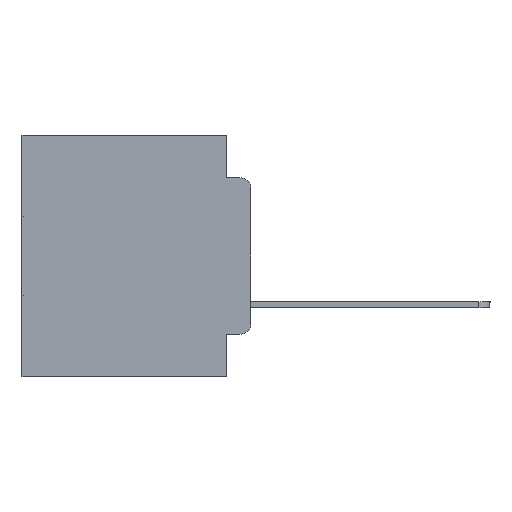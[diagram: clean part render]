
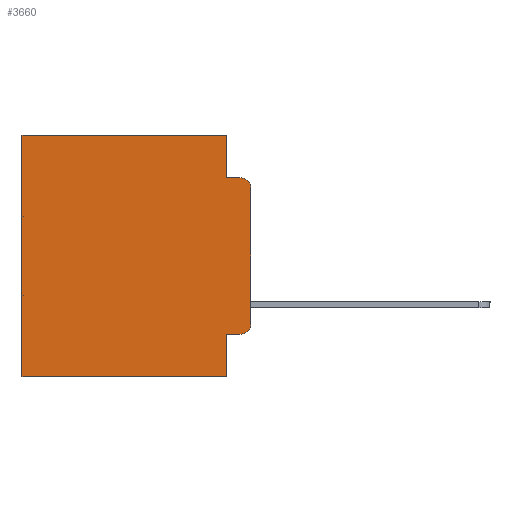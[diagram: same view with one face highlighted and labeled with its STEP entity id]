
A CAD part, left-side view. The second image highlights one B-rep face of the part: STEP entity #3660.
In plain terms, the highlighted planar face has unit normal (-1, 0, 0).
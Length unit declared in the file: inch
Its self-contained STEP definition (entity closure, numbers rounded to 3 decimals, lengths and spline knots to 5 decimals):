
#218 = DIRECTION ( 'NONE',  ( 0., -1., 0. ) ) ;
#1203 = EDGE_CURVE ( 'NONE', #16348, #26457, #9020, .T. ) ;
#1427 = FACE_OUTER_BOUND ( 'NONE', #21408, .T. ) ;
#1746 = VERTEX_POINT ( 'NONE', #16600 ) ;
#1847 = CARTESIAN_POINT ( 'NONE',  ( 0.298, 0.473, 0. ) ) ;
#1998 = ORIENTED_EDGE ( 'NONE', *, *, #12314, .T. ) ;
#2050 = PLANE ( 'NONE',  #3455 ) ;
#2650 = VERTEX_POINT ( 'NONE', #5294 ) ;
#2804 = VECTOR ( 'NONE', #5925, 39.37008 ) ;
#3455 = AXIS2_PLACEMENT_3D ( 'NONE', #23412, #21355, #13927 ) ;
#3605 = DIRECTION ( 'NONE',  ( -1., 0., 0. ) ) ;
#3660 = ADVANCED_FACE ( 'NONE', ( #1427 ), #2050, .F. ) ;
#5294 = CARTESIAN_POINT ( 'NONE',  ( 0.298, 0.02, -0.0885 ) ) ;
#5925 = DIRECTION ( 'NONE',  ( 0., 0., -1. ) ) ;
#5948 = DIRECTION ( 'NONE',  ( -1., 0., 0. ) ) ;
#6258 = DIRECTION ( 'NONE',  ( 0., 0., -1. ) ) ;
#6486 = EDGE_CURVE ( 'NONE', #21719, #12941, #17036, .T. ) ;
#6664 = EDGE_CURVE ( 'NONE', #25098, #12713, #27475, .T. ) ;
#7265 = ORIENTED_EDGE ( 'NONE', *, *, #10635, .F. ) ;
#8189 = ORIENTED_EDGE ( 'NONE', *, *, #6664, .F. ) ;
#8225 = ORIENTED_EDGE ( 'NONE', *, *, #14018, .T. ) ;
#8260 = LINE ( 'NONE', #17913, #14005 ) ;
#8399 = CARTESIAN_POINT ( 'NONE',  ( 0.298, 0.051, 0. ) ) ;
#8950 = CARTESIAN_POINT ( 'NONE',  ( 0.298, 0.02, -0.1085 ) ) ;
#9020 = LINE ( 'NONE', #8399, #13879 ) ;
#9315 = ORIENTED_EDGE ( 'NONE', *, *, #1203, .F. ) ;
#9660 = LINE ( 'NONE', #28969, #24577 ) ;
#10124 = EDGE_CURVE ( 'NONE', #18295, #1746, #8260, .T. ) ;
#10198 = VERTEX_POINT ( 'NONE', #21042 ) ;
#10420 = AXIS2_PLACEMENT_3D ( 'NONE', #15810, #3605, #25456 ) ;
#10635 = EDGE_CURVE ( 'NONE', #26457, #12941, #21210, .T. ) ;
#10666 = CARTESIAN_POINT ( 'NONE',  ( 0.298, 0.051, 0. ) ) ;
#11536 = VECTOR ( 'NONE', #17351, 39.37008 ) ;
#11693 = CARTESIAN_POINT ( 'NONE',  ( 0.298, 0., -0.5 ) ) ;
#11803 = DIRECTION ( 'NONE',  ( 0., 0., -1. ) ) ;
#12004 = ORIENTED_EDGE ( 'NONE', *, *, #31243, .F. ) ;
#12314 = EDGE_CURVE ( 'NONE', #10198, #1746, #20119, .T. ) ;
#12427 = LINE ( 'NONE', #22096, #11536 ) ;
#12503 = ORIENTED_EDGE ( 'NONE', *, *, #10124, .F. ) ;
#12713 = VERTEX_POINT ( 'NONE', #15618 ) ;
#12941 = VERTEX_POINT ( 'NONE', #16563 ) ;
#13879 = VECTOR ( 'NONE', #25955, 39.37008 ) ;
#13927 = DIRECTION ( 'NONE',  ( 0., 0., -1. ) ) ;
#14005 = VECTOR ( 'NONE', #15704, 39.37008 ) ;
#14018 = EDGE_CURVE ( 'NONE', #18295, #2650, #20139, .T. ) ;
#14651 = CARTESIAN_POINT ( 'NONE',  ( 0.298, 0.051, -0.0885 ) ) ;
#15618 = CARTESIAN_POINT ( 'NONE',  ( 0.298, 0.051, -0.0885 ) ) ;
#15704 = DIRECTION ( 'NONE',  ( 0., 0., -1. ) ) ;
#15810 = CARTESIAN_POINT ( 'NONE',  ( 0.298, 0.02, -0.3915 ) ) ;
#16348 = VERTEX_POINT ( 'NONE', #23513 ) ;
#16563 = CARTESIAN_POINT ( 'NONE',  ( 0.298, 0.473, -0.5 ) ) ;
#16600 = CARTESIAN_POINT ( 'NONE',  ( 0.298, 0., -0.3915 ) ) ;
#16622 = VECTOR ( 'NONE', #218, 39.37008 ) ;
#17036 = LINE ( 'NONE', #1847, #17962 ) ;
#17154 = CARTESIAN_POINT ( 'NONE',  ( 0.298, 0., -0.1085 ) ) ;
#17351 = DIRECTION ( 'NONE',  ( 0., -1., 0. ) ) ;
#17738 = DIRECTION ( 'NONE',  ( 0., 1., 0. ) ) ;
#17913 = CARTESIAN_POINT ( 'NONE',  ( 0.298, 0., 0. ) ) ;
#17962 = VECTOR ( 'NONE', #11803, 39.37008 ) ;
#18295 = VERTEX_POINT ( 'NONE', #17154 ) ;
#18346 = ORIENTED_EDGE ( 'NONE', *, *, #22167, .T. ) ;
#19289 = CARTESIAN_POINT ( 'NONE',  ( 0.298, 0.051, -0.5 ) ) ;
#19649 = ORIENTED_EDGE ( 'NONE', *, *, #6486, .T. ) ;
#20119 = CIRCLE ( 'NONE', #10420, 0.02 ) ;
#20139 = CIRCLE ( 'NONE', #22679, 0.02 ) ;
#21042 = CARTESIAN_POINT ( 'NONE',  ( 0.298, 0.02, -0.4115 ) ) ;
#21210 = LINE ( 'NONE', #11693, #21569 ) ;
#21355 = DIRECTION ( 'NONE',  ( 1., 0., 0. ) ) ;
#21408 = EDGE_LOOP ( 'NONE', ( #12503, #8225, #12004, #8189, #18346, #19649, #7265, #9315, #29201, #1998 ) ) ;
#21569 = VECTOR ( 'NONE', #30879, 39.37008 ) ;
#21719 = VERTEX_POINT ( 'NONE', #29966 ) ;
#22096 = CARTESIAN_POINT ( 'NONE',  ( 0.298, 0.051, -0.4115 ) ) ;
#22167 = EDGE_CURVE ( 'NONE', #25098, #21719, #9660, .T. ) ;
#22679 = AXIS2_PLACEMENT_3D ( 'NONE', #8950, #5948, #6258 ) ;
#23412 = CARTESIAN_POINT ( 'NONE',  ( 0.298, 0., 0. ) ) ;
#23513 = CARTESIAN_POINT ( 'NONE',  ( 0.298, 0.051, -0.4115 ) ) ;
#23656 = CARTESIAN_POINT ( 'NONE',  ( 0.298, 0.051, 0. ) ) ;
#24577 = VECTOR ( 'NONE', #17738, 39.37008 ) ;
#25098 = VERTEX_POINT ( 'NONE', #23656 ) ;
#25456 = DIRECTION ( 'NONE',  ( 0., 0., -1. ) ) ;
#25955 = DIRECTION ( 'NONE',  ( 0., 0., -1. ) ) ;
#26002 = EDGE_CURVE ( 'NONE', #16348, #10198, #12427, .T. ) ;
#26457 = VERTEX_POINT ( 'NONE', #19289 ) ;
#26653 = LINE ( 'NONE', #14651, #16622 ) ;
#27475 = LINE ( 'NONE', #10666, #2804 ) ;
#28969 = CARTESIAN_POINT ( 'NONE',  ( 0.298, 0., 0. ) ) ;
#29201 = ORIENTED_EDGE ( 'NONE', *, *, #26002, .T. ) ;
#29966 = CARTESIAN_POINT ( 'NONE',  ( 0.298, 0.473, 0. ) ) ;
#30879 = DIRECTION ( 'NONE',  ( 0., 1., 0. ) ) ;
#31243 = EDGE_CURVE ( 'NONE', #12713, #2650, #26653, .T. ) ;
